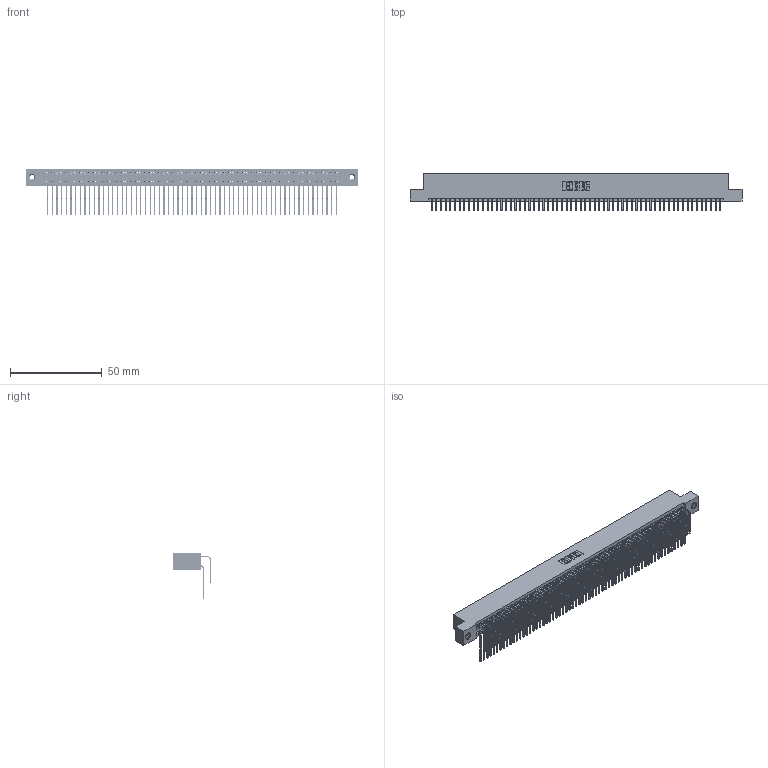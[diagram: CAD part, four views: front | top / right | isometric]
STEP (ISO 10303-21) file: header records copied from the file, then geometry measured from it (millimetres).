
FILE_DESCRIPTION (( 'STEP AP203' ), '1' );
FILE_NAME ('345-126-559-207.STEP', '2018-10-19T17:57:06', ( '' ), ( '' ), 'SwSTEP 2.0', 'SolidWorks 2016', '' );
FILE_SCHEMA (( 'CONFIG_CONTROL_DESIGN' ));
Length unit declared in the file: inch
Products named in the file (5): 345-126-559-207; 345-292-001_559 Tail - 2; 345-292-001_558 559 Tail - 1; 345-250-001_345-250-005-103; 345 Part_Flush Mounting Lugs - 0.156 Dia-TI
Assembly tree (129 placements, depth 2):
  345-126-559-207
    345 Part_Flush Mounting Lugs - 0.156 Dia-TI
    345-292-001_558 559 Tail - 1  x63
    345-292-001_559 Tail - 2  x63
    345-250-001_345-250-005-103  x2
Bounding box: 181.23 x 20.56 x 25.53 mm (x, y, z)
Volume: 18513 mm3; surface area: 31217.9 mm2
Topology: 129 solids, 129 shells, 6738 faces, 20007 edges, 13162 vertices
Faces by surface type: plane 4522, cylinder 2200, cone 12, torus 4
Entity records: 49442 total; most frequent: CARTESIAN_POINT 8294, ORIENTED_EDGE 8170, DIRECTION 7287, EDGE_CURVE 4085, VECTOR 3641, LINE 3641, VERTEX_POINT 2716, AXIS2_PLACEMENT_3D 1823
